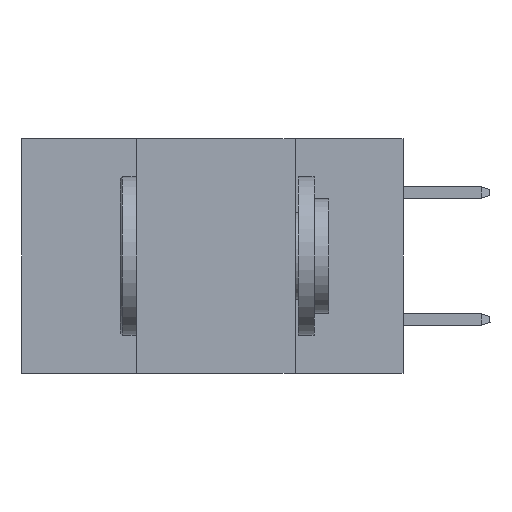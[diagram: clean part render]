
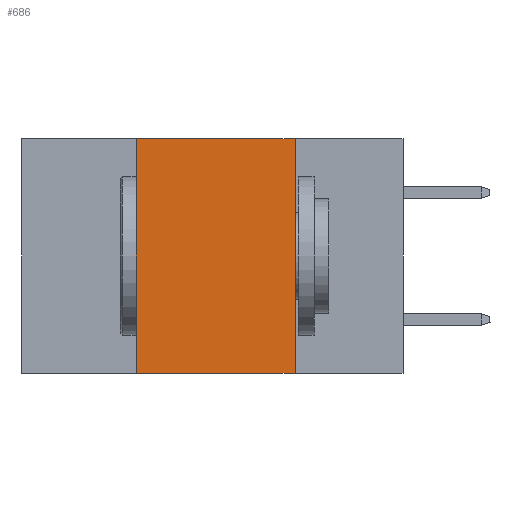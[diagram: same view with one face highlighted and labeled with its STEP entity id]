
A CAD part, left-side view. The second image highlights one B-rep face of the part: STEP entity #686.
In plain terms, the highlighted planar face has unit normal (-1, 0, 0).
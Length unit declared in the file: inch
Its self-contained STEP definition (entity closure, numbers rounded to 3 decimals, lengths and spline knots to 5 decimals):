
#352 = CARTESIAN_POINT ( 'NONE',  ( 0., 0.42, -0.37 ) ) ;
#686 = ADVANCED_FACE ( 'NONE', ( #11309 ), #7616, .F. ) ;
#969 = VECTOR ( 'NONE', #1970, 39.37008 ) ;
#1053 = DIRECTION ( 'NONE',  ( 0., -1., 0. ) ) ;
#1417 = VERTEX_POINT ( 'NONE', #8814 ) ;
#1590 = ORIENTED_EDGE ( 'NONE', *, *, #10237, .F. ) ;
#1970 = DIRECTION ( 'NONE',  ( 0., -1., 0. ) ) ;
#2708 = AXIS2_PLACEMENT_3D ( 'NONE', #3487, #13922, #15388 ) ;
#2709 = CARTESIAN_POINT ( 'NONE',  ( 0., 0.17, 0. ) ) ;
#3220 = VERTEX_POINT ( 'NONE', #16031 ) ;
#3487 = CARTESIAN_POINT ( 'NONE',  ( 0., 0.6, 0. ) ) ;
#3516 = CARTESIAN_POINT ( 'NONE',  ( 0., 0.6, -0.37 ) ) ;
#4474 = DIRECTION ( 'NONE',  ( 0., 0., 1. ) ) ;
#4849 = ORIENTED_EDGE ( 'NONE', *, *, #14001, .T. ) ;
#5979 = ORIENTED_EDGE ( 'NONE', *, *, #7444, .F. ) ;
#7444 = EDGE_CURVE ( 'NONE', #3220, #10000, #9231, .T. ) ;
#7563 = CARTESIAN_POINT ( 'NONE',  ( 0., 0.6, 0. ) ) ;
#7616 = PLANE ( 'NONE',  #2708 ) ;
#7960 = DIRECTION ( 'NONE',  ( 0., 0., -1. ) ) ;
#8259 = CARTESIAN_POINT ( 'NONE',  ( 0., 0.42, 0. ) ) ;
#8508 = LINE ( 'NONE', #3516, #969 ) ;
#8814 = CARTESIAN_POINT ( 'NONE',  ( 0., 0.42, 0. ) ) ;
#9082 = VECTOR ( 'NONE', #7960, 39.37008 ) ;
#9086 = EDGE_LOOP ( 'NONE', ( #5979, #15371, #1590, #4849 ) ) ;
#9231 = LINE ( 'NONE', #2709, #9082 ) ;
#9674 = VECTOR ( 'NONE', #1053, 39.37008 ) ;
#10000 = VERTEX_POINT ( 'NONE', #13143 ) ;
#10237 = EDGE_CURVE ( 'NONE', #13915, #1417, #15934, .T. ) ;
#10381 = VECTOR ( 'NONE', #4474, 39.37008 ) ;
#11309 = FACE_OUTER_BOUND ( 'NONE', #9086, .T. ) ;
#13143 = CARTESIAN_POINT ( 'NONE',  ( 0., 0.17, -0.37 ) ) ;
#13446 = EDGE_CURVE ( 'NONE', #1417, #3220, #14059, .T. ) ;
#13915 = VERTEX_POINT ( 'NONE', #352 ) ;
#13922 = DIRECTION ( 'NONE',  ( 1., 0., 0. ) ) ;
#14001 = EDGE_CURVE ( 'NONE', #13915, #10000, #8508, .T. ) ;
#14059 = LINE ( 'NONE', #7563, #9674 ) ;
#15371 = ORIENTED_EDGE ( 'NONE', *, *, #13446, .F. ) ;
#15388 = DIRECTION ( 'NONE',  ( 0., 0., -1. ) ) ;
#15934 = LINE ( 'NONE', #8259, #10381 ) ;
#16031 = CARTESIAN_POINT ( 'NONE',  ( 0., 0.17, 0. ) ) ;
